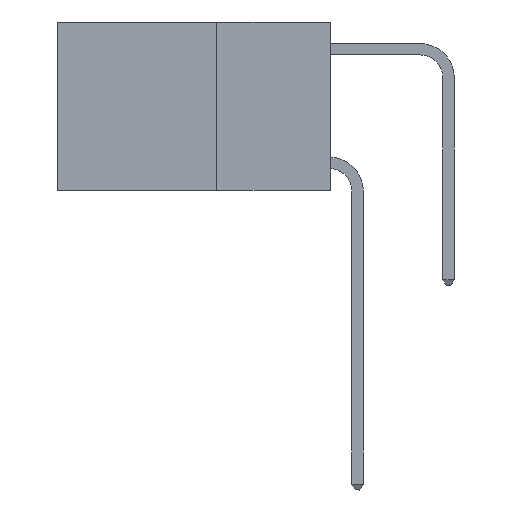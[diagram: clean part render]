
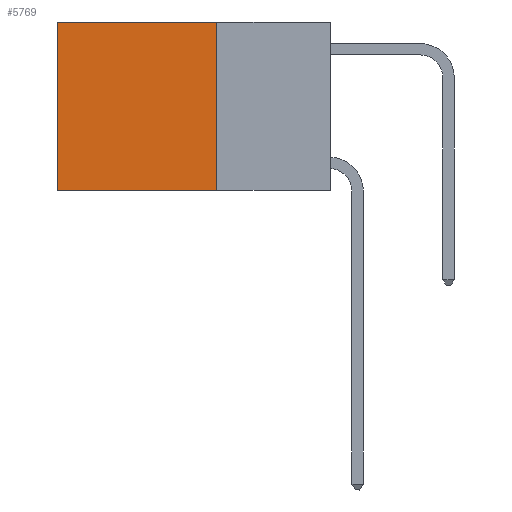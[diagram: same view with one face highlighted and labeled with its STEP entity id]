
A CAD part, left-side view. The second image highlights one B-rep face of the part: STEP entity #5769.
In plain terms, the highlighted planar face has unit normal (-1, 0, 0).
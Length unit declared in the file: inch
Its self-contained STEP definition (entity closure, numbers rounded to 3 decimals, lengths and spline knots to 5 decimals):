
#287 = CARTESIAN_POINT ( 'NONE',  ( 0.2625, 0.6, 0. ) ) ;
#316 = DIRECTION ( 'NONE',  ( 0., 0., -1. ) ) ;
#429 = CARTESIAN_POINT ( 'NONE',  ( 0.2625, 0.25, 0. ) ) ;
#652 = EDGE_CURVE ( 'NONE', #6351, #11762, #3012, .T. ) ;
#965 = EDGE_CURVE ( 'NONE', #8968, #11762, #7891, .T. ) ;
#1585 = DIRECTION ( 'NONE',  ( 0., 0., -1. ) ) ;
#1693 = CARTESIAN_POINT ( 'NONE',  ( 0.2625, 0.6, 0. ) ) ;
#1994 = VECTOR ( 'NONE', #316, 39.37008 ) ;
#2258 = VECTOR ( 'NONE', #7729, 39.37008 ) ;
#2637 = FACE_OUTER_BOUND ( 'NONE', #7772, .T. ) ;
#2662 = VECTOR ( 'NONE', #13239, 39.37008 ) ;
#3012 = LINE ( 'NONE', #6385, #2662 ) ;
#3846 = LINE ( 'NONE', #8653, #6319 ) ;
#4962 = EDGE_CURVE ( 'NONE', #5440, #8968, #3846, .T. ) ;
#5440 = VERTEX_POINT ( 'NONE', #5445 ) ;
#5445 = CARTESIAN_POINT ( 'NONE',  ( 0.2625, 0.25, 0. ) ) ;
#5630 = DIRECTION ( 'NONE',  ( 0., 1., 0. ) ) ;
#5769 = ADVANCED_FACE ( 'NONE', ( #2637 ), #9843, .F. ) ;
#6319 = VECTOR ( 'NONE', #5630, 39.37008 ) ;
#6351 = VERTEX_POINT ( 'NONE', #10432 ) ;
#6385 = CARTESIAN_POINT ( 'NONE',  ( 0.2625, 0.25, -0.37 ) ) ;
#7729 = DIRECTION ( 'NONE',  ( 0., 0., -1. ) ) ;
#7772 = EDGE_LOOP ( 'NONE', ( #10810, #13270, #10026, #12943 ) ) ;
#7831 = LINE ( 'NONE', #11673, #2258 ) ;
#7871 = DIRECTION ( 'NONE',  ( 1., 0., 0. ) ) ;
#7891 = LINE ( 'NONE', #287, #1994 ) ;
#8137 = EDGE_CURVE ( 'NONE', #5440, #6351, #7831, .T. ) ;
#8653 = CARTESIAN_POINT ( 'NONE',  ( 0.2625, 0.25, 0. ) ) ;
#8968 = VERTEX_POINT ( 'NONE', #1693 ) ;
#9843 = PLANE ( 'NONE',  #10309 ) ;
#10026 = ORIENTED_EDGE ( 'NONE', *, *, #8137, .F. ) ;
#10309 = AXIS2_PLACEMENT_3D ( 'NONE', #429, #7871, #1585 ) ;
#10432 = CARTESIAN_POINT ( 'NONE',  ( 0.2625, 0.25, -0.37 ) ) ;
#10810 = ORIENTED_EDGE ( 'NONE', *, *, #965, .T. ) ;
#11673 = CARTESIAN_POINT ( 'NONE',  ( 0.2625, 0.25, 0. ) ) ;
#11762 = VERTEX_POINT ( 'NONE', #12184 ) ;
#12184 = CARTESIAN_POINT ( 'NONE',  ( 0.2625, 0.6, -0.37 ) ) ;
#12943 = ORIENTED_EDGE ( 'NONE', *, *, #4962, .T. ) ;
#13239 = DIRECTION ( 'NONE',  ( 0., 1., 0. ) ) ;
#13270 = ORIENTED_EDGE ( 'NONE', *, *, #652, .F. ) ;
